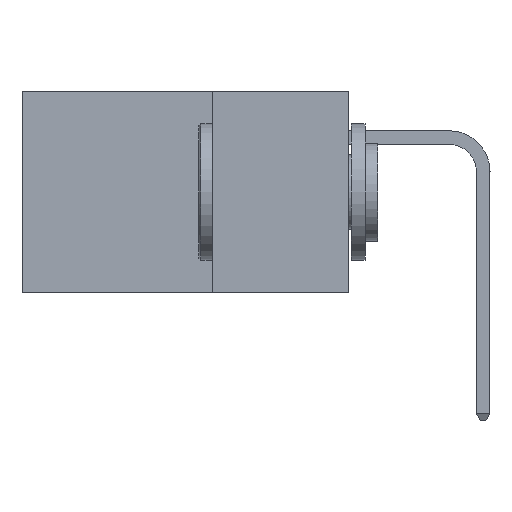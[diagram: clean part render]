
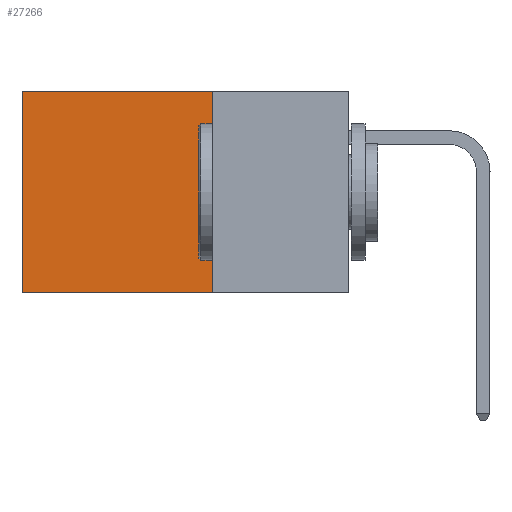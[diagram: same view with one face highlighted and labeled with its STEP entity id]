
A CAD part, left-side view. The second image highlights one B-rep face of the part: STEP entity #27266.
In plain terms, the highlighted planar face has unit normal (-1, 0, 0).
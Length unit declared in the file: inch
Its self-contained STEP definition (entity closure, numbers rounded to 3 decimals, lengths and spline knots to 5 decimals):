
#637 = DIRECTION ( 'NONE',  ( 0., 0., -1. ) ) ;
#4499 = VECTOR ( 'NONE', #13760, 39.37008 ) ;
#4969 = ORIENTED_EDGE ( 'NONE', *, *, #7035, .T. ) ;
#5760 = ORIENTED_EDGE ( 'NONE', *, *, #19864, .F. ) ;
#6658 = VERTEX_POINT ( 'NONE', #20130 ) ;
#6675 = CARTESIAN_POINT ( 'NONE',  ( 0.2875, 0.25, 0. ) ) ;
#7035 = EDGE_CURVE ( 'NONE', #22969, #27910, #38772, .T. ) ;
#7405 = DIRECTION ( 'NONE',  ( 0., 1., 0. ) ) ;
#8532 = VECTOR ( 'NONE', #9856, 39.37008 ) ;
#9856 = DIRECTION ( 'NONE',  ( 0., 1., 0. ) ) ;
#10194 = PLANE ( 'NONE',  #37392 ) ;
#10543 = CARTESIAN_POINT ( 'NONE',  ( 0.2875, 0.25, 0. ) ) ;
#10856 = CARTESIAN_POINT ( 'NONE',  ( 0.2875, 0.6, 0. ) ) ;
#13262 = EDGE_LOOP ( 'NONE', ( #4969, #13570, #5760, #20626 ) ) ;
#13570 = ORIENTED_EDGE ( 'NONE', *, *, #27316, .F. ) ;
#13724 = EDGE_CURVE ( 'NONE', #18381, #22969, #33557, .T. ) ;
#13760 = DIRECTION ( 'NONE',  ( 0., 0., -1. ) ) ;
#13925 = VECTOR ( 'NONE', #14081, 39.37008 ) ;
#14081 = DIRECTION ( 'NONE',  ( 0., 0., -1. ) ) ;
#15710 = FACE_OUTER_BOUND ( 'NONE', #13262, .T. ) ;
#18381 = VERTEX_POINT ( 'NONE', #10543 ) ;
#19597 = CARTESIAN_POINT ( 'NONE',  ( 0.2875, 0.6, -0.37 ) ) ;
#19769 = DIRECTION ( 'NONE',  ( 1., 0., 0. ) ) ;
#19864 = EDGE_CURVE ( 'NONE', #18381, #6658, #38272, .T. ) ;
#20130 = CARTESIAN_POINT ( 'NONE',  ( 0.2875, 0.25, -0.37 ) ) ;
#20626 = ORIENTED_EDGE ( 'NONE', *, *, #13724, .T. ) ;
#22969 = VERTEX_POINT ( 'NONE', #30412 ) ;
#23202 = CARTESIAN_POINT ( 'NONE',  ( 0.2875, 0.25, -0.37 ) ) ;
#27266 = ADVANCED_FACE ( 'NONE', ( #15710 ), #10194, .F. ) ;
#27316 = EDGE_CURVE ( 'NONE', #6658, #27910, #38552, .T. ) ;
#27910 = VERTEX_POINT ( 'NONE', #19597 ) ;
#30412 = CARTESIAN_POINT ( 'NONE',  ( 0.2875, 0.6, 0. ) ) ;
#33557 = LINE ( 'NONE', #6675, #8532 ) ;
#35472 = CARTESIAN_POINT ( 'NONE',  ( 0.2875, 0.25, 0. ) ) ;
#37392 = AXIS2_PLACEMENT_3D ( 'NONE', #38339, #19769, #637 ) ;
#37605 = VECTOR ( 'NONE', #7405, 39.37008 ) ;
#38272 = LINE ( 'NONE', #35472, #4499 ) ;
#38339 = CARTESIAN_POINT ( 'NONE',  ( 0.2875, 0.25, 0. ) ) ;
#38552 = LINE ( 'NONE', #23202, #37605 ) ;
#38772 = LINE ( 'NONE', #10856, #13925 ) ;
